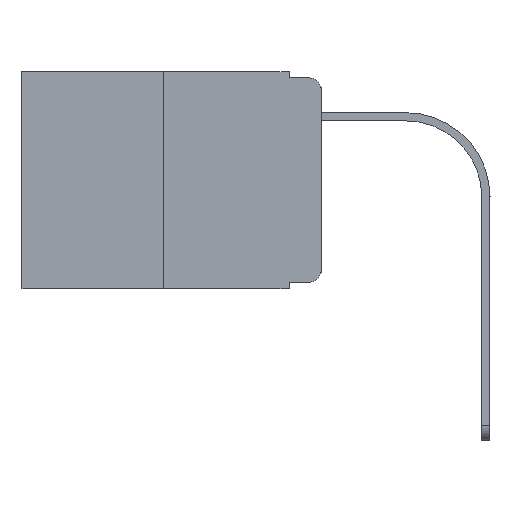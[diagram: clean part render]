
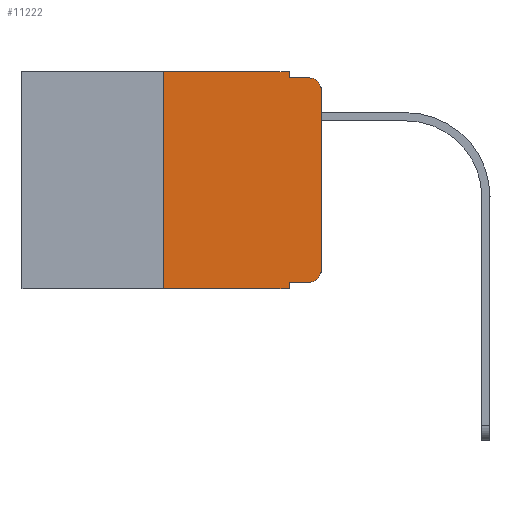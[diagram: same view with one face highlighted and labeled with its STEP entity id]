
A CAD part, left-side view. The second image highlights one B-rep face of the part: STEP entity #11222.
In plain terms, the highlighted planar face has unit normal (-1, 0, 0).
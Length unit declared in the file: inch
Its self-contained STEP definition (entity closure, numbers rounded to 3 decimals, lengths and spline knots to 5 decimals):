
#41 = LINE ( 'NONE', #11781, #9790 ) ;
#342 = VERTEX_POINT ( 'NONE', #4855 ) ;
#487 = CARTESIAN_POINT ( 'NONE',  ( 0., 0.051, -0.333 ) ) ;
#668 = CARTESIAN_POINT ( 'NONE',  ( 0., 0.473, 0. ) ) ;
#861 = CARTESIAN_POINT ( 'NONE',  ( 0., 0.473, -0.343 ) ) ;
#910 = CARTESIAN_POINT ( 'NONE',  ( 0., 0.473, 0. ) ) ;
#928 = LINE ( 'NONE', #10060, #3769 ) ;
#1423 = LINE ( 'NONE', #2631, #5323 ) ;
#1713 = LINE ( 'NONE', #487, #15183 ) ;
#1912 = VECTOR ( 'NONE', #19044, 39.37008 ) ;
#2182 = DIRECTION ( 'NONE',  ( 0., 0., -1. ) ) ;
#2333 = CARTESIAN_POINT ( 'NONE',  ( 0., 0.051, -0.343 ) ) ;
#2631 = CARTESIAN_POINT ( 'NONE',  ( 0., 0.051, -0.01 ) ) ;
#2744 = CARTESIAN_POINT ( 'NONE',  ( 0., 0.051, 0. ) ) ;
#3235 = CARTESIAN_POINT ( 'NONE',  ( 0., 0.02, -0.03 ) ) ;
#3361 = VECTOR ( 'NONE', #5455, 39.37008 ) ;
#3769 = VECTOR ( 'NONE', #12960, 39.37008 ) ;
#4108 = EDGE_CURVE ( 'NONE', #17498, #8068, #1713, .T. ) ;
#4651 = EDGE_CURVE ( 'NONE', #4936, #10724, #18950, .T. ) ;
#4855 = CARTESIAN_POINT ( 'NONE',  ( 0., 0.25, 0. ) ) ;
#4936 = VERTEX_POINT ( 'NONE', #10880 ) ;
#5030 = AXIS2_PLACEMENT_3D ( 'NONE', #3235, #15363, #6514 ) ;
#5232 = ORIENTED_EDGE ( 'NONE', *, *, #10265, .F. ) ;
#5240 = AXIS2_PLACEMENT_3D ( 'NONE', #6663, #9725, #2182 ) ;
#5323 = VECTOR ( 'NONE', #16343, 39.37008 ) ;
#5415 = ORIENTED_EDGE ( 'NONE', *, *, #8214, .F. ) ;
#5455 = DIRECTION ( 'NONE',  ( 0., -1., 0. ) ) ;
#5484 = EDGE_CURVE ( 'NONE', #14563, #15013, #14633, .T. ) ;
#6265 = VERTEX_POINT ( 'NONE', #12410 ) ;
#6445 = CARTESIAN_POINT ( 'NONE',  ( 0., 0., -0.313 ) ) ;
#6514 = DIRECTION ( 'NONE',  ( 0., 0., -1. ) ) ;
#6663 = CARTESIAN_POINT ( 'NONE',  ( 0., 0.02, -0.313 ) ) ;
#6728 = VERTEX_POINT ( 'NONE', #6445 ) ;
#7136 = CARTESIAN_POINT ( 'NONE',  ( 0., 0.02, -0.333 ) ) ;
#7170 = EDGE_CURVE ( 'NONE', #4936, #342, #7370, .T. ) ;
#7370 = LINE ( 'NONE', #11161, #16160 ) ;
#7782 = CIRCLE ( 'NONE', #5240, 0.02 ) ;
#8068 = VERTEX_POINT ( 'NONE', #7136 ) ;
#8214 = EDGE_CURVE ( 'NONE', #17498, #10724, #41, .T. ) ;
#8336 = CARTESIAN_POINT ( 'NONE',  ( 0., 0.051, -0.333 ) ) ;
#8403 = EDGE_CURVE ( 'NONE', #12318, #6265, #17726, .T. ) ;
#8462 = FACE_OUTER_BOUND ( 'NONE', #19387, .T. ) ;
#8479 = EDGE_CURVE ( 'NONE', #6728, #12318, #928, .T. ) ;
#9175 = ORIENTED_EDGE ( 'NONE', *, *, #8479, .T. ) ;
#9725 = DIRECTION ( 'NONE',  ( -1., 0., 0. ) ) ;
#9790 = VECTOR ( 'NONE', #14864, 39.37008 ) ;
#10060 = CARTESIAN_POINT ( 'NONE',  ( 0., 0., 0. ) ) ;
#10228 = DIRECTION ( 'NONE',  ( 0., 0., 1. ) ) ;
#10257 = ORIENTED_EDGE ( 'NONE', *, *, #13288, .F. ) ;
#10265 = EDGE_CURVE ( 'NONE', #342, #14563, #17173, .T. ) ;
#10370 = VECTOR ( 'NONE', #13051, 39.37008 ) ;
#10563 = CARTESIAN_POINT ( 'NONE',  ( 0., 0.051, -0.01 ) ) ;
#10724 = VERTEX_POINT ( 'NONE', #2333 ) ;
#10787 = ORIENTED_EDGE ( 'NONE', *, *, #18540, .T. ) ;
#10880 = CARTESIAN_POINT ( 'NONE',  ( 0., 0.25, -0.343 ) ) ;
#11161 = CARTESIAN_POINT ( 'NONE',  ( 0., 0.25, 0. ) ) ;
#11222 = ADVANCED_FACE ( 'NONE', ( #8462 ), #14527, .F. ) ;
#11257 = ORIENTED_EDGE ( 'NONE', *, *, #5484, .F. ) ;
#11781 = CARTESIAN_POINT ( 'NONE',  ( 0., 0.051, 0. ) ) ;
#12318 = VERTEX_POINT ( 'NONE', #14437 ) ;
#12410 = CARTESIAN_POINT ( 'NONE',  ( 0., 0.02, -0.01 ) ) ;
#12960 = DIRECTION ( 'NONE',  ( 0., 0., 1. ) ) ;
#13051 = DIRECTION ( 'NONE',  ( 0., 0., -1. ) ) ;
#13288 = EDGE_CURVE ( 'NONE', #15013, #6265, #1423, .T. ) ;
#13379 = AXIS2_PLACEMENT_3D ( 'NONE', #910, #19094, #17611 ) ;
#14361 = ORIENTED_EDGE ( 'NONE', *, *, #4108, .T. ) ;
#14437 = CARTESIAN_POINT ( 'NONE',  ( 0., 0., -0.03 ) ) ;
#14520 = ORIENTED_EDGE ( 'NONE', *, *, #8403, .T. ) ;
#14527 = PLANE ( 'NONE',  #13379 ) ;
#14563 = VERTEX_POINT ( 'NONE', #2744 ) ;
#14633 = LINE ( 'NONE', #16023, #10370 ) ;
#14864 = DIRECTION ( 'NONE',  ( 0., 0., -1. ) ) ;
#15013 = VERTEX_POINT ( 'NONE', #10563 ) ;
#15105 = ORIENTED_EDGE ( 'NONE', *, *, #4651, .T. ) ;
#15183 = VECTOR ( 'NONE', #19601, 39.37008 ) ;
#15363 = DIRECTION ( 'NONE',  ( -1., 0., 0. ) ) ;
#16023 = CARTESIAN_POINT ( 'NONE',  ( 0., 0.051, 0. ) ) ;
#16160 = VECTOR ( 'NONE', #10228, 39.37008 ) ;
#16343 = DIRECTION ( 'NONE',  ( 0., -1., 0. ) ) ;
#17173 = LINE ( 'NONE', #668, #1912 ) ;
#17498 = VERTEX_POINT ( 'NONE', #8336 ) ;
#17611 = DIRECTION ( 'NONE',  ( 0., 0., -1. ) ) ;
#17726 = CIRCLE ( 'NONE', #5030, 0.02 ) ;
#18294 = ORIENTED_EDGE ( 'NONE', *, *, #7170, .F. ) ;
#18540 = EDGE_CURVE ( 'NONE', #8068, #6728, #7782, .T. ) ;
#18950 = LINE ( 'NONE', #861, #3361 ) ;
#19044 = DIRECTION ( 'NONE',  ( 0., -1., 0. ) ) ;
#19094 = DIRECTION ( 'NONE',  ( 1., 0., 0. ) ) ;
#19387 = EDGE_LOOP ( 'NONE', ( #9175, #14520, #10257, #11257, #5232, #18294, #15105, #5415, #14361, #10787 ) ) ;
#19601 = DIRECTION ( 'NONE',  ( 0., -1., 0. ) ) ;
